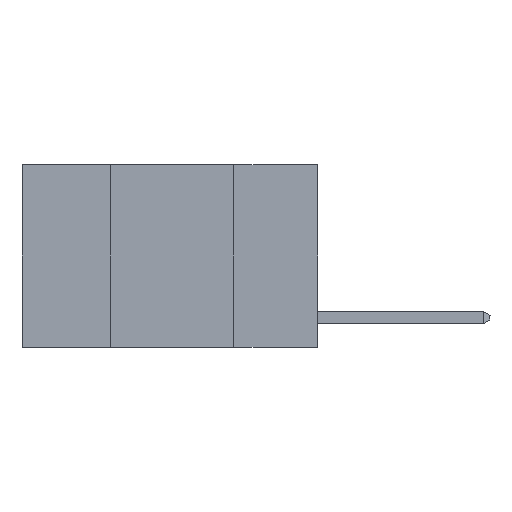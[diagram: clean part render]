
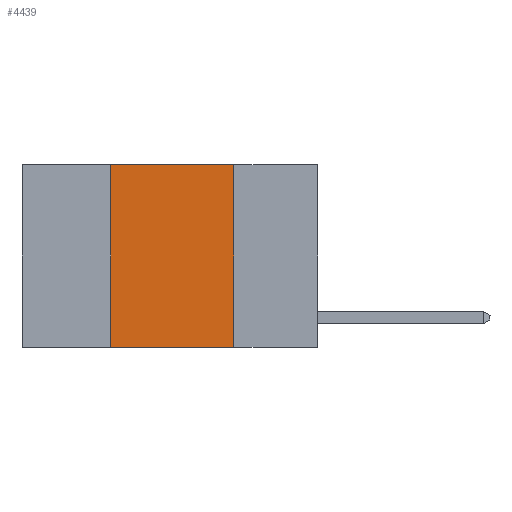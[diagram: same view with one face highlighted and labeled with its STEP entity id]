
A CAD part, left-side view. The second image highlights one B-rep face of the part: STEP entity #4439.
In plain terms, the highlighted planar face has unit normal (-1, 0, 0).
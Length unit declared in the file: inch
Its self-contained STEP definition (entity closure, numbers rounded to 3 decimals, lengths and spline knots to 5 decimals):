
#15 = DIRECTION ( 'NONE',  ( 1., 0., 0. ) ) ;
#1980 = EDGE_LOOP ( 'NONE', ( #10376, #3394, #15935, #3683 ) ) ;
#2153 = LINE ( 'NONE', #8289, #11055 ) ;
#2488 = FACE_OUTER_BOUND ( 'NONE', #1980, .T. ) ;
#3394 = ORIENTED_EDGE ( 'NONE', *, *, #7582, .F. ) ;
#3683 = ORIENTED_EDGE ( 'NONE', *, *, #9512, .T. ) ;
#3810 = VECTOR ( 'NONE', #9232, 39.37008 ) ;
#3813 = CARTESIAN_POINT ( 'NONE',  ( 0., 0.17, 0. ) ) ;
#4364 = CARTESIAN_POINT ( 'NONE',  ( 0., 0.17, -0.37 ) ) ;
#4439 = ADVANCED_FACE ( 'NONE', ( #2488 ), #7555, .F. ) ;
#4895 = CARTESIAN_POINT ( 'NONE',  ( 0., 0.17, 0. ) ) ;
#6310 = CARTESIAN_POINT ( 'NONE',  ( 0., 0.6, 0. ) ) ;
#6835 = LINE ( 'NONE', #11918, #15107 ) ;
#6974 = DIRECTION ( 'NONE',  ( 0., -1., 0. ) ) ;
#7555 = PLANE ( 'NONE',  #10231 ) ;
#7582 = EDGE_CURVE ( 'NONE', #9793, #7906, #9059, .T. ) ;
#7906 = VERTEX_POINT ( 'NONE', #4895 ) ;
#8289 = CARTESIAN_POINT ( 'NONE',  ( 0., 0.6, -0.37 ) ) ;
#8412 = CARTESIAN_POINT ( 'NONE',  ( 0., 0.42, -0.37 ) ) ;
#9059 = LINE ( 'NONE', #14174, #3810 ) ;
#9105 = CARTESIAN_POINT ( 'NONE',  ( 0., 0.42, 0. ) ) ;
#9232 = DIRECTION ( 'NONE',  ( 0., -1., 0. ) ) ;
#9512 = EDGE_CURVE ( 'NONE', #11714, #15282, #2153, .T. ) ;
#9793 = VERTEX_POINT ( 'NONE', #9105 ) ;
#10231 = AXIS2_PLACEMENT_3D ( 'NONE', #6310, #15, #11484 ) ;
#10376 = ORIENTED_EDGE ( 'NONE', *, *, #15538, .F. ) ;
#11055 = VECTOR ( 'NONE', #6974, 39.37008 ) ;
#11086 = DIRECTION ( 'NONE',  ( 0., 0., -1. ) ) ;
#11484 = DIRECTION ( 'NONE',  ( 0., 0., -1. ) ) ;
#11714 = VERTEX_POINT ( 'NONE', #8412 ) ;
#11918 = CARTESIAN_POINT ( 'NONE',  ( 0., 0.42, 0. ) ) ;
#13251 = EDGE_CURVE ( 'NONE', #11714, #9793, #6835, .T. ) ;
#13303 = VECTOR ( 'NONE', #11086, 39.37008 ) ;
#14174 = CARTESIAN_POINT ( 'NONE',  ( 0., 0.6, 0. ) ) ;
#14515 = DIRECTION ( 'NONE',  ( 0., 0., 1. ) ) ;
#15107 = VECTOR ( 'NONE', #14515, 39.37008 ) ;
#15244 = LINE ( 'NONE', #3813, #13303 ) ;
#15282 = VERTEX_POINT ( 'NONE', #4364 ) ;
#15538 = EDGE_CURVE ( 'NONE', #7906, #15282, #15244, .T. ) ;
#15935 = ORIENTED_EDGE ( 'NONE', *, *, #13251, .F. ) ;
